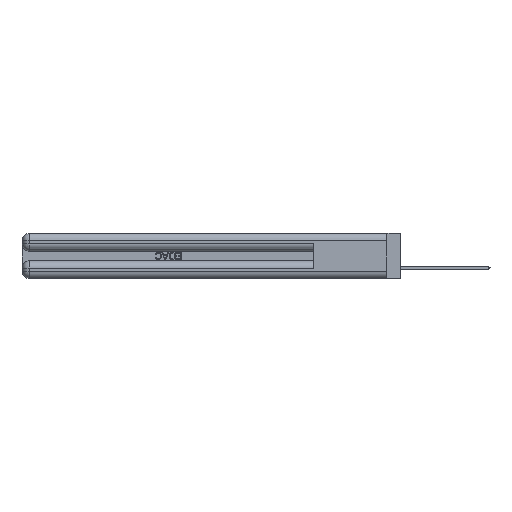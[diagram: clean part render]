
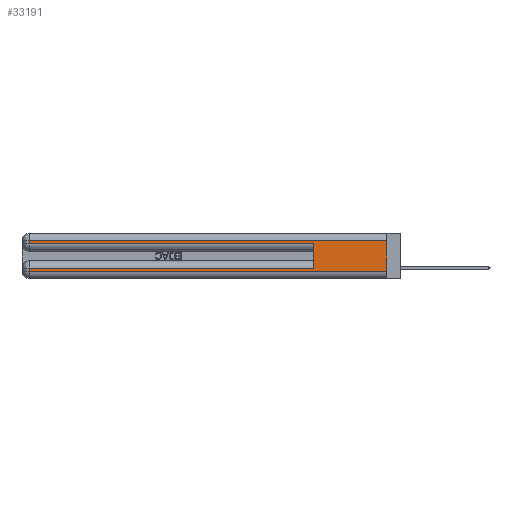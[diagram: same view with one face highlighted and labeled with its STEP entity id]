
A CAD part, left-side view. The second image highlights one B-rep face of the part: STEP entity #33191.
In plain terms, the highlighted planar face has unit normal (-1, 0, 0).
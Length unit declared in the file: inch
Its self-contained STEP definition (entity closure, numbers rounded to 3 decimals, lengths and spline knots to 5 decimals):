
#769 = DIRECTION ( 'NONE',  ( 0., 0., -1. ) ) ;
#1085 = CARTESIAN_POINT ( 'NONE',  ( 0., 2.94, 0.37 ) ) ;
#1590 = CARTESIAN_POINT ( 'NONE',  ( 0., 2.94, 0.06 ) ) ;
#1661 = CARTESIAN_POINT ( 'NONE',  ( 0., 2.94, 0.31 ) ) ;
#2266 = CARTESIAN_POINT ( 'NONE',  ( 0., 2.94, 0.285 ) ) ;
#2561 = ORIENTED_EDGE ( 'NONE', *, *, #18840, .F. ) ;
#2593 = EDGE_CURVE ( 'NONE', #3333, #10892, #37454, .T. ) ;
#3321 = ORIENTED_EDGE ( 'NONE', *, *, #42795, .T. ) ;
#3333 = VERTEX_POINT ( 'NONE', #34161 ) ;
#3973 = LINE ( 'NONE', #10502, #31148 ) ;
#5290 = CARTESIAN_POINT ( 'NONE',  ( 0., 0.6, 0.285 ) ) ;
#6611 = EDGE_CURVE ( 'NONE', #34850, #20479, #12022, .T. ) ;
#9209 = DIRECTION ( 'NONE',  ( 0., 1., 0. ) ) ;
#9743 = ORIENTED_EDGE ( 'NONE', *, *, #6611, .T. ) ;
#10502 = CARTESIAN_POINT ( 'NONE',  ( 0., 0., 0.06 ) ) ;
#10892 = VERTEX_POINT ( 'NONE', #33484 ) ;
#10894 = PLANE ( 'NONE',  #34522 ) ;
#11395 = VECTOR ( 'NONE', #9209, 39.37008 ) ;
#11835 = CARTESIAN_POINT ( 'NONE',  ( 0., 0., 0.31 ) ) ;
#12022 = LINE ( 'NONE', #44860, #11395 ) ;
#12272 = VECTOR ( 'NONE', #24678, 39.37008 ) ;
#12825 = DIRECTION ( 'NONE',  ( 0., 0., -1. ) ) ;
#13199 = VERTEX_POINT ( 'NONE', #1590 ) ;
#13469 = DIRECTION ( 'NONE',  ( 0., 0., -1. ) ) ;
#14004 = CARTESIAN_POINT ( 'NONE',  ( 0., 0., 0.285 ) ) ;
#15065 = CARTESIAN_POINT ( 'NONE',  ( 0., 0., 0.37 ) ) ;
#15932 = ORIENTED_EDGE ( 'NONE', *, *, #29071, .T. ) ;
#18016 = LINE ( 'NONE', #11835, #12272 ) ;
#18840 = EDGE_CURVE ( 'NONE', #34850, #39069, #25074, .T. ) ;
#18953 = CARTESIAN_POINT ( 'NONE',  ( 0., 2.94, 0.085 ) ) ;
#19265 = DIRECTION ( 'NONE',  ( 1., 0., 0. ) ) ;
#20479 = VERTEX_POINT ( 'NONE', #18953 ) ;
#21512 = FACE_OUTER_BOUND ( 'NONE', #36420, .T. ) ;
#21659 = CARTESIAN_POINT ( 'NONE',  ( 0., 2.94, 0.37 ) ) ;
#22073 = CARTESIAN_POINT ( 'NONE',  ( 0., 0.6, 0.085 ) ) ;
#23852 = VECTOR ( 'NONE', #13469, 39.37008 ) ;
#23896 = VECTOR ( 'NONE', #769, 39.37008 ) ;
#24347 = CARTESIAN_POINT ( 'NONE',  ( 0., 0.6, 0.145 ) ) ;
#24678 = DIRECTION ( 'NONE',  ( 0., 1., 0. ) ) ;
#25074 = LINE ( 'NONE', #24347, #49650 ) ;
#26801 = LINE ( 'NONE', #14004, #41754 ) ;
#28882 = DIRECTION ( 'NONE',  ( 0., 0., 1. ) ) ;
#29071 = EDGE_CURVE ( 'NONE', #13199, #10892, #3973, .T. ) ;
#31148 = VECTOR ( 'NONE', #52753, 39.37008 ) ;
#31960 = VERTEX_POINT ( 'NONE', #2266 ) ;
#32767 = EDGE_CURVE ( 'NONE', #31960, #39069, #26801, .T. ) ;
#33191 = ADVANCED_FACE ( 'NONE', ( #21512 ), #10894, .F. ) ;
#33484 = CARTESIAN_POINT ( 'NONE',  ( 0., 0., 0.06 ) ) ;
#34161 = CARTESIAN_POINT ( 'NONE',  ( 0., 0., 0.31 ) ) ;
#34522 = AXIS2_PLACEMENT_3D ( 'NONE', #15065, #19265, #35357 ) ;
#34850 = VERTEX_POINT ( 'NONE', #22073 ) ;
#35357 = DIRECTION ( 'NONE',  ( 0., 0., -1. ) ) ;
#36124 = EDGE_CURVE ( 'NONE', #3333, #39649, #18016, .T. ) ;
#36420 = EDGE_LOOP ( 'NONE', ( #46217, #48844, #52104, #47037, #2561, #9743, #3321, #15932 ) ) ;
#36731 = CARTESIAN_POINT ( 'NONE',  ( 0., 0., 0.37 ) ) ;
#36874 = LINE ( 'NONE', #1085, #23852 ) ;
#36954 = EDGE_CURVE ( 'NONE', #39649, #31960, #36874, .T. ) ;
#37454 = LINE ( 'NONE', #36731, #49085 ) ;
#39069 = VERTEX_POINT ( 'NONE', #5290 ) ;
#39649 = VERTEX_POINT ( 'NONE', #1661 ) ;
#40110 = LINE ( 'NONE', #21659, #23896 ) ;
#41754 = VECTOR ( 'NONE', #51465, 39.37008 ) ;
#42795 = EDGE_CURVE ( 'NONE', #20479, #13199, #40110, .T. ) ;
#44860 = CARTESIAN_POINT ( 'NONE',  ( 0., 0., 0.085 ) ) ;
#46217 = ORIENTED_EDGE ( 'NONE', *, *, #2593, .F. ) ;
#47037 = ORIENTED_EDGE ( 'NONE', *, *, #32767, .T. ) ;
#48844 = ORIENTED_EDGE ( 'NONE', *, *, #36124, .T. ) ;
#49085 = VECTOR ( 'NONE', #12825, 39.37008 ) ;
#49650 = VECTOR ( 'NONE', #28882, 39.37008 ) ;
#51465 = DIRECTION ( 'NONE',  ( 0., -1., 0. ) ) ;
#52104 = ORIENTED_EDGE ( 'NONE', *, *, #36954, .T. ) ;
#52753 = DIRECTION ( 'NONE',  ( 0., -1., 0. ) ) ;
